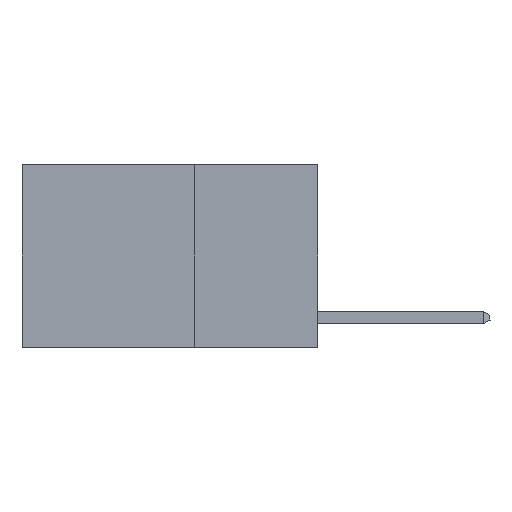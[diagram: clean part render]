
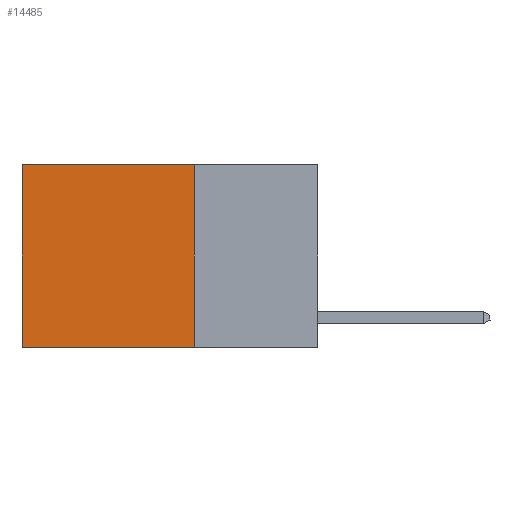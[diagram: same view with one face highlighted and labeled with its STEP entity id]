
A CAD part, left-side view. The second image highlights one B-rep face of the part: STEP entity #14485.
In plain terms, the highlighted planar face has unit normal (-1, 0, 0).
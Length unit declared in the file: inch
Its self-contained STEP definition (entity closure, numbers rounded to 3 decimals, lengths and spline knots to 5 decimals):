
#195 = VECTOR ( 'NONE', #452, 39.37008 ) ;
#452 = DIRECTION ( 'NONE',  ( 0., 0., -1. ) ) ;
#2598 = CARTESIAN_POINT ( 'NONE',  ( 0.2625, 0.25, 0. ) ) ;
#2941 = DIRECTION ( 'NONE',  ( 0., 0., -1. ) ) ;
#3244 = VERTEX_POINT ( 'NONE', #18924 ) ;
#3639 = EDGE_LOOP ( 'NONE', ( #13047, #12720, #8387, #11731 ) ) ;
#4091 = DIRECTION ( 'NONE',  ( 1., 0., 0. ) ) ;
#5016 = CARTESIAN_POINT ( 'NONE',  ( 0.2625, 0.25, -0.37 ) ) ;
#5914 = VECTOR ( 'NONE', #16566, 39.37008 ) ;
#6301 = VECTOR ( 'NONE', #2941, 39.37008 ) ;
#6361 = CARTESIAN_POINT ( 'NONE',  ( 0.2625, 0.25, 0. ) ) ;
#7279 = EDGE_CURVE ( 'NONE', #10307, #3244, #17946, .T. ) ;
#8169 = EDGE_CURVE ( 'NONE', #3244, #15540, #10162, .T. ) ;
#8387 = ORIENTED_EDGE ( 'NONE', *, *, #7279, .F. ) ;
#8428 = FACE_OUTER_BOUND ( 'NONE', #3639, .T. ) ;
#8655 = EDGE_CURVE ( 'NONE', #10307, #18350, #9807, .T. ) ;
#9698 = VECTOR ( 'NONE', #13771, 39.37008 ) ;
#9807 = LINE ( 'NONE', #6361, #5914 ) ;
#10162 = LINE ( 'NONE', #5016, #9698 ) ;
#10286 = CARTESIAN_POINT ( 'NONE',  ( 0.2625, 0.6, 0. ) ) ;
#10307 = VERTEX_POINT ( 'NONE', #10461 ) ;
#10461 = CARTESIAN_POINT ( 'NONE',  ( 0.2625, 0.25, 0. ) ) ;
#11398 = PLANE ( 'NONE',  #14998 ) ;
#11731 = ORIENTED_EDGE ( 'NONE', *, *, #8655, .T. ) ;
#11947 = LINE ( 'NONE', #18023, #195 ) ;
#12720 = ORIENTED_EDGE ( 'NONE', *, *, #8169, .F. ) ;
#13047 = ORIENTED_EDGE ( 'NONE', *, *, #17406, .T. ) ;
#13174 = CARTESIAN_POINT ( 'NONE',  ( 0.2625, 0.25, 0. ) ) ;
#13771 = DIRECTION ( 'NONE',  ( 0., 1., 0. ) ) ;
#14325 = DIRECTION ( 'NONE',  ( 0., 0., -1. ) ) ;
#14485 = ADVANCED_FACE ( 'NONE', ( #8428 ), #11398, .F. ) ;
#14998 = AXIS2_PLACEMENT_3D ( 'NONE', #2598, #4091, #14325 ) ;
#15540 = VERTEX_POINT ( 'NONE', #16640 ) ;
#16566 = DIRECTION ( 'NONE',  ( 0., 1., 0. ) ) ;
#16640 = CARTESIAN_POINT ( 'NONE',  ( 0.2625, 0.6, -0.37 ) ) ;
#17406 = EDGE_CURVE ( 'NONE', #18350, #15540, #11947, .T. ) ;
#17946 = LINE ( 'NONE', #13174, #6301 ) ;
#18023 = CARTESIAN_POINT ( 'NONE',  ( 0.2625, 0.6, 0. ) ) ;
#18350 = VERTEX_POINT ( 'NONE', #10286 ) ;
#18924 = CARTESIAN_POINT ( 'NONE',  ( 0.2625, 0.25, -0.37 ) ) ;
